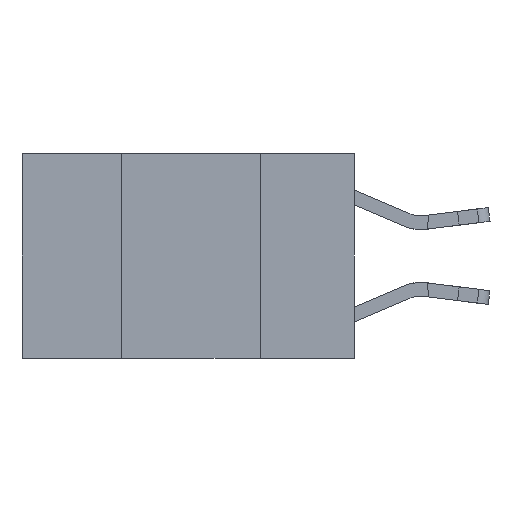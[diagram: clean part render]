
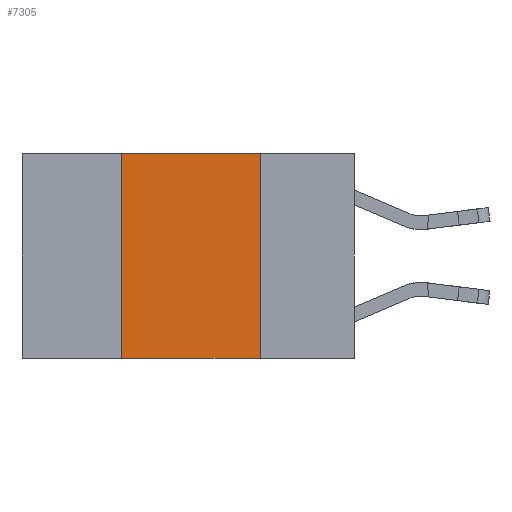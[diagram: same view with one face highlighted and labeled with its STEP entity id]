
A CAD part, left-side view. The second image highlights one B-rep face of the part: STEP entity #7305.
In plain terms, the highlighted planar face has unit normal (-1, 0, 0).
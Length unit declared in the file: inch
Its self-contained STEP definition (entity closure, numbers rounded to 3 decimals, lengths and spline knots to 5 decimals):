
#36 = AXIS2_PLACEMENT_3D ( 'NONE', #15348, #7813, #3870 ) ;
#47 = LINE ( 'NONE', #11222, #10461 ) ;
#167 = CARTESIAN_POINT ( 'NONE',  ( 0., 0.42, 0. ) ) ;
#329 = EDGE_CURVE ( 'NONE', #10691, #4356, #1495, .T. ) ;
#441 = CARTESIAN_POINT ( 'NONE',  ( 0., 0.17, 0. ) ) ;
#1195 = EDGE_CURVE ( 'NONE', #2481, #9011, #8419, .T. ) ;
#1228 = ORIENTED_EDGE ( 'NONE', *, *, #1195, .F. ) ;
#1495 = LINE ( 'NONE', #167, #11082 ) ;
#2085 = DIRECTION ( 'NONE',  ( 0., -1., 0. ) ) ;
#2481 = VERTEX_POINT ( 'NONE', #441 ) ;
#3870 = DIRECTION ( 'NONE',  ( 0., 0., -1. ) ) ;
#4356 = VERTEX_POINT ( 'NONE', #7979 ) ;
#5145 = ORIENTED_EDGE ( 'NONE', *, *, #12193, .F. ) ;
#6566 = CARTESIAN_POINT ( 'NONE',  ( 0., 0.42, -0.37 ) ) ;
#6970 = CARTESIAN_POINT ( 'NONE',  ( 0., 0.17, -0.37 ) ) ;
#7107 = DIRECTION ( 'NONE',  ( 0., 0., -1. ) ) ;
#7305 = ADVANCED_FACE ( 'NONE', ( #9674 ), #11422, .F. ) ;
#7813 = DIRECTION ( 'NONE',  ( 1., 0., 0. ) ) ;
#7979 = CARTESIAN_POINT ( 'NONE',  ( 0., 0.42, 0. ) ) ;
#8419 = LINE ( 'NONE', #8628, #12228 ) ;
#8597 = ORIENTED_EDGE ( 'NONE', *, *, #329, .F. ) ;
#8628 = CARTESIAN_POINT ( 'NONE',  ( 0., 0.17, 0. ) ) ;
#8941 = DIRECTION ( 'NONE',  ( 0., -1., 0. ) ) ;
#9011 = VERTEX_POINT ( 'NONE', #6970 ) ;
#9191 = ORIENTED_EDGE ( 'NONE', *, *, #16042, .T. ) ;
#9674 = FACE_OUTER_BOUND ( 'NONE', #16047, .T. ) ;
#10461 = VECTOR ( 'NONE', #2085, 39.37008 ) ;
#10691 = VERTEX_POINT ( 'NONE', #6566 ) ;
#11082 = VECTOR ( 'NONE', #13425, 39.37008 ) ;
#11222 = CARTESIAN_POINT ( 'NONE',  ( 0., 0.6, -0.37 ) ) ;
#11377 = VECTOR ( 'NONE', #8941, 39.37008 ) ;
#11422 = PLANE ( 'NONE',  #36 ) ;
#12193 = EDGE_CURVE ( 'NONE', #4356, #2481, #13930, .T. ) ;
#12228 = VECTOR ( 'NONE', #7107, 39.37008 ) ;
#13425 = DIRECTION ( 'NONE',  ( 0., 0., 1. ) ) ;
#13930 = LINE ( 'NONE', #14013, #11377 ) ;
#14013 = CARTESIAN_POINT ( 'NONE',  ( 0., 0.6, 0. ) ) ;
#15348 = CARTESIAN_POINT ( 'NONE',  ( 0., 0.6, 0. ) ) ;
#16042 = EDGE_CURVE ( 'NONE', #10691, #9011, #47, .T. ) ;
#16047 = EDGE_LOOP ( 'NONE', ( #1228, #5145, #8597, #9191 ) ) ;
